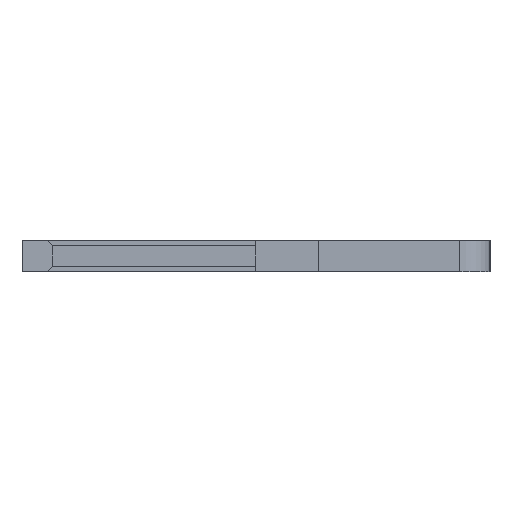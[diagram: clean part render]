
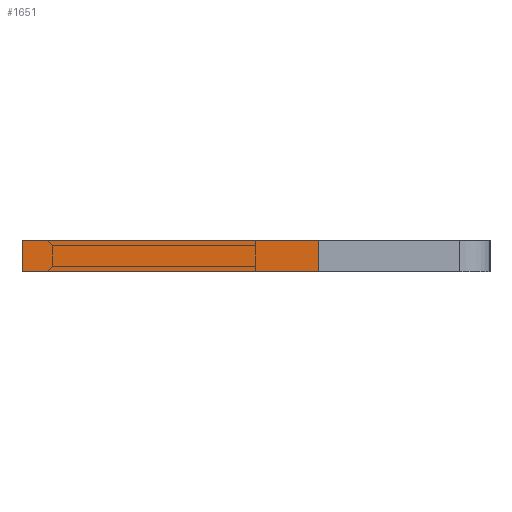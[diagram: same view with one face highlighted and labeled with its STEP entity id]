
A CAD part, left-side view. The second image highlights one B-rep face of the part: STEP entity #1651.
In plain terms, the highlighted face is planar.
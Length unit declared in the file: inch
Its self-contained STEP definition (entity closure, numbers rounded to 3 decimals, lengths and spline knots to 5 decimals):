
#50 = DIRECTION ( 'NONE',  ( 0., 0., 1. ) ) ;
#71 = AXIS2_PLACEMENT_3D ( 'NONE', #440, #50, #251 ) ;
#82 = CARTESIAN_POINT ( 'NONE',  ( -0.01, 0.15, -0.04 ) ) ;
#180 = CARTESIAN_POINT ( 'NONE',  ( 0.01, 0.15, -0.04 ) ) ;
#229 = ORIENTED_EDGE ( 'NONE', *, *, #942, .T. ) ;
#251 = DIRECTION ( 'NONE',  ( 1., 0., 0. ) ) ;
#416 = LINE ( 'NONE', #2089, #1792 ) ;
#440 = CARTESIAN_POINT ( 'NONE',  ( 0.01, 0.15, -0.04 ) ) ;
#550 = DIRECTION ( 'NONE',  ( -1., 0., 0. ) ) ;
#601 = EDGE_LOOP ( 'NONE', ( #2134, #1299, #781, #229 ) ) ;
#730 = VECTOR ( 'NONE', #1935, 39.37008 ) ;
#781 = ORIENTED_EDGE ( 'NONE', *, *, #1239, .F. ) ;
#862 = CARTESIAN_POINT ( 'NONE',  ( -0.01, 0.15, -0.04 ) ) ;
#942 = EDGE_CURVE ( 'NONE', #1543, #1608, #416, .T. ) ;
#992 = CARTESIAN_POINT ( 'NONE',  ( 0.01, 0.15, -0.04 ) ) ;
#1098 = EDGE_CURVE ( 'NONE', #2046, #1670, #1740, .T. ) ;
#1124 = LINE ( 'NONE', #862, #1679 ) ;
#1230 = DIRECTION ( 'NONE',  ( 0., 1., 0. ) ) ;
#1239 = EDGE_CURVE ( 'NONE', #1543, #2046, #2207, .T. ) ;
#1247 = CARTESIAN_POINT ( 'NONE',  ( 0.01, 0.15, -0.04 ) ) ;
#1299 = ORIENTED_EDGE ( 'NONE', *, *, #1098, .F. ) ;
#1379 = CARTESIAN_POINT ( 'NONE',  ( 0.01, -0.04, -0.04 ) ) ;
#1391 = PLANE ( 'NONE',  #71 ) ;
#1543 = VERTEX_POINT ( 'NONE', #1379 ) ;
#1608 = VERTEX_POINT ( 'NONE', #1751 ) ;
#1618 = FACE_OUTER_BOUND ( 'NONE', #601, .T. ) ;
#1651 = ADVANCED_FACE ( 'NONE', ( #1618 ), #1391, .F. ) ;
#1670 = VERTEX_POINT ( 'NONE', #82 ) ;
#1679 = VECTOR ( 'NONE', #1230, 39.37008 ) ;
#1692 = DIRECTION ( 'NONE',  ( -1., 0., 0. ) ) ;
#1740 = LINE ( 'NONE', #180, #1849 ) ;
#1751 = CARTESIAN_POINT ( 'NONE',  ( -0.01, -0.04, -0.04 ) ) ;
#1792 = VECTOR ( 'NONE', #550, 39.37008 ) ;
#1849 = VECTOR ( 'NONE', #1692, 39.37008 ) ;
#1935 = DIRECTION ( 'NONE',  ( 0., 1., 0. ) ) ;
#2046 = VERTEX_POINT ( 'NONE', #1247 ) ;
#2089 = CARTESIAN_POINT ( 'NONE',  ( 0.01, -0.04, -0.04 ) ) ;
#2111 = EDGE_CURVE ( 'NONE', #1608, #1670, #1124, .T. ) ;
#2134 = ORIENTED_EDGE ( 'NONE', *, *, #2111, .T. ) ;
#2207 = LINE ( 'NONE', #992, #730 ) ;
